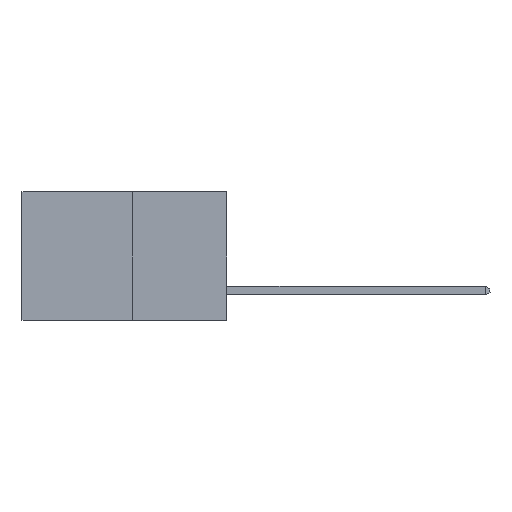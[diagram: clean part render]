
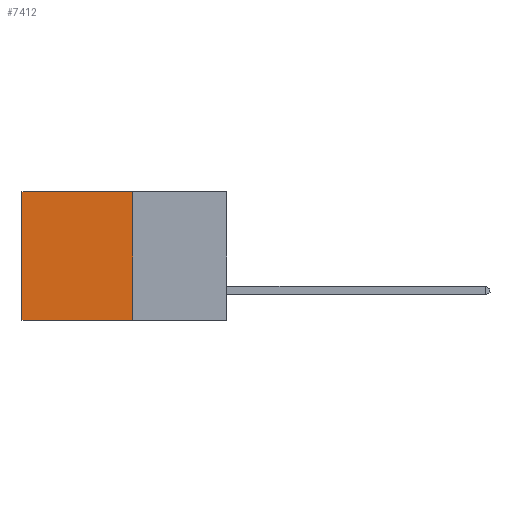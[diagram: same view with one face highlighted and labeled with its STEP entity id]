
A CAD part, left-side view. The second image highlights one B-rep face of the part: STEP entity #7412.
In plain terms, the highlighted planar face has unit normal (-1, 0, 0).
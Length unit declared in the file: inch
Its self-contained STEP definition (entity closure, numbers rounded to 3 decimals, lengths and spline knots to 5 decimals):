
#214 = EDGE_CURVE ( 'NONE', #5692, #7641, #6477, .T. ) ;
#789 = PLANE ( 'NONE',  #6065 ) ;
#871 = LINE ( 'NONE', #2022, #2801 ) ;
#886 = DIRECTION ( 'NONE',  ( 0., 0., -1. ) ) ;
#1255 = CARTESIAN_POINT ( 'NONE',  ( 0.277, 0.59, -0.37 ) ) ;
#1684 = DIRECTION ( 'NONE',  ( 0., 1., 0. ) ) ;
#1803 = VECTOR ( 'NONE', #2166, 39.37008 ) ;
#2022 = CARTESIAN_POINT ( 'NONE',  ( 0.277, 0.27, -0.37 ) ) ;
#2166 = DIRECTION ( 'NONE',  ( 0., 0., -1. ) ) ;
#2213 = CARTESIAN_POINT ( 'NONE',  ( 0.277, 0.27, 0. ) ) ;
#2214 = VECTOR ( 'NONE', #3903, 39.37008 ) ;
#2270 = EDGE_LOOP ( 'NONE', ( #5762, #5687, #5706, #4744 ) ) ;
#2801 = VECTOR ( 'NONE', #886, 39.37008 ) ;
#2867 = CARTESIAN_POINT ( 'NONE',  ( 0.277, 0.27, -0.37 ) ) ;
#2938 = DIRECTION ( 'NONE',  ( 0., 0., -1. ) ) ;
#2992 = DIRECTION ( 'NONE',  ( 1., 0., 0. ) ) ;
#3217 = CARTESIAN_POINT ( 'NONE',  ( 0.277, 0.27, -0.37 ) ) ;
#3302 = CARTESIAN_POINT ( 'NONE',  ( 0.277, 0.59, -0.37 ) ) ;
#3650 = LINE ( 'NONE', #1255, #1803 ) ;
#3903 = DIRECTION ( 'NONE',  ( 0., 1., 0. ) ) ;
#4258 = LINE ( 'NONE', #2213, #2214 ) ;
#4541 = EDGE_CURVE ( 'NONE', #5592, #5692, #871, .T. ) ;
#4744 = ORIENTED_EDGE ( 'NONE', *, *, #7919, .T. ) ;
#5530 = CARTESIAN_POINT ( 'NONE',  ( 0.277, 0.59, 0. ) ) ;
#5592 = VERTEX_POINT ( 'NONE', #6114 ) ;
#5687 = ORIENTED_EDGE ( 'NONE', *, *, #214, .F. ) ;
#5692 = VERTEX_POINT ( 'NONE', #8209 ) ;
#5706 = ORIENTED_EDGE ( 'NONE', *, *, #4541, .F. ) ;
#5762 = ORIENTED_EDGE ( 'NONE', *, *, #7573, .T. ) ;
#6065 = AXIS2_PLACEMENT_3D ( 'NONE', #3217, #2992, #2938 ) ;
#6114 = CARTESIAN_POINT ( 'NONE',  ( 0.277, 0.27, 0. ) ) ;
#6231 = VERTEX_POINT ( 'NONE', #5530 ) ;
#6477 = LINE ( 'NONE', #2867, #8007 ) ;
#7412 = ADVANCED_FACE ( 'NONE', ( #8320 ), #789, .F. ) ;
#7573 = EDGE_CURVE ( 'NONE', #6231, #7641, #3650, .T. ) ;
#7641 = VERTEX_POINT ( 'NONE', #3302 ) ;
#7919 = EDGE_CURVE ( 'NONE', #5592, #6231, #4258, .T. ) ;
#8007 = VECTOR ( 'NONE', #1684, 39.37008 ) ;
#8209 = CARTESIAN_POINT ( 'NONE',  ( 0.277, 0.27, -0.37 ) ) ;
#8320 = FACE_OUTER_BOUND ( 'NONE', #2270, .T. ) ;
